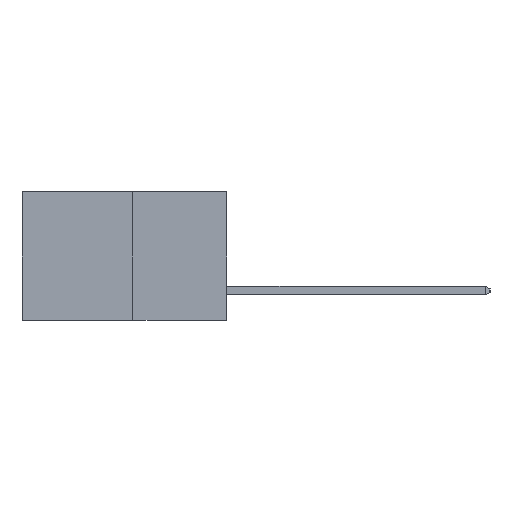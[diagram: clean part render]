
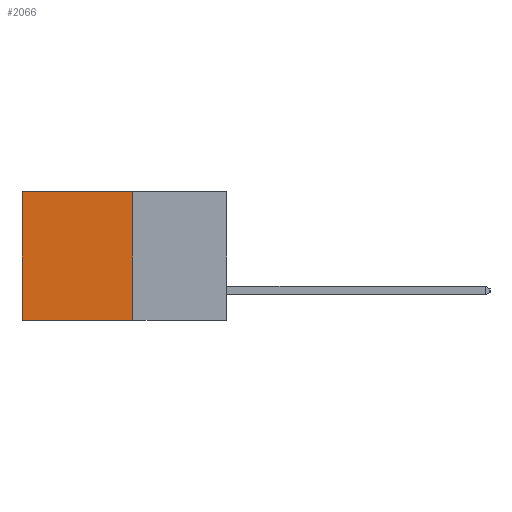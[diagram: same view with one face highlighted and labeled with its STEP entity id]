
A CAD part, left-side view. The second image highlights one B-rep face of the part: STEP entity #2066.
In plain terms, the highlighted planar face has unit normal (-1, 0, 0).
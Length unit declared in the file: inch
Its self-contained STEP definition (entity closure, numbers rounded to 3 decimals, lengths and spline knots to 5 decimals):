
#570 = VERTEX_POINT ( 'NONE', #11419 ) ;
#684 = EDGE_CURVE ( 'NONE', #3620, #5594, #8739, .T. ) ;
#844 = VECTOR ( 'NONE', #13764, 39.37008 ) ;
#1901 = PLANE ( 'NONE',  #9061 ) ;
#2066 = ADVANCED_FACE ( 'NONE', ( #10842 ), #1901, .F. ) ;
#2217 = EDGE_LOOP ( 'NONE', ( #8002, #12167, #5767, #13775 ) ) ;
#2970 = VERTEX_POINT ( 'NONE', #7666 ) ;
#3016 = EDGE_CURVE ( 'NONE', #570, #5594, #9937, .T. ) ;
#3083 = VECTOR ( 'NONE', #10998, 39.37008 ) ;
#3231 = CARTESIAN_POINT ( 'NONE',  ( 0.277, 0.27, 0. ) ) ;
#3547 = DIRECTION ( 'NONE',  ( 0., 0., -1. ) ) ;
#3620 = VERTEX_POINT ( 'NONE', #4545 ) ;
#3797 = LINE ( 'NONE', #3231, #12473 ) ;
#4545 = CARTESIAN_POINT ( 'NONE',  ( 0.277, 0.27, -0.37 ) ) ;
#4642 = LINE ( 'NONE', #8030, #844 ) ;
#5428 = EDGE_CURVE ( 'NONE', #2970, #570, #3797, .T. ) ;
#5594 = VERTEX_POINT ( 'NONE', #9767 ) ;
#5767 = ORIENTED_EDGE ( 'NONE', *, *, #13887, .F. ) ;
#7078 = DIRECTION ( 'NONE',  ( 0., 0., -1. ) ) ;
#7666 = CARTESIAN_POINT ( 'NONE',  ( 0.277, 0.27, 0. ) ) ;
#8002 = ORIENTED_EDGE ( 'NONE', *, *, #3016, .T. ) ;
#8030 = CARTESIAN_POINT ( 'NONE',  ( 0.277, 0.27, -0.37 ) ) ;
#8093 = CARTESIAN_POINT ( 'NONE',  ( 0.277, 0.27, -0.37 ) ) ;
#8477 = CARTESIAN_POINT ( 'NONE',  ( 0.277, 0.59, -0.37 ) ) ;
#8739 = LINE ( 'NONE', #8093, #3083 ) ;
#8903 = DIRECTION ( 'NONE',  ( 0., 1., 0. ) ) ;
#9061 = AXIS2_PLACEMENT_3D ( 'NONE', #13373, #11158, #3547 ) ;
#9567 = VECTOR ( 'NONE', #7078, 39.37008 ) ;
#9767 = CARTESIAN_POINT ( 'NONE',  ( 0.277, 0.59, -0.37 ) ) ;
#9937 = LINE ( 'NONE', #8477, #9567 ) ;
#10842 = FACE_OUTER_BOUND ( 'NONE', #2217, .T. ) ;
#10998 = DIRECTION ( 'NONE',  ( 0., 1., 0. ) ) ;
#11158 = DIRECTION ( 'NONE',  ( 1., 0., 0. ) ) ;
#11419 = CARTESIAN_POINT ( 'NONE',  ( 0.277, 0.59, 0. ) ) ;
#12167 = ORIENTED_EDGE ( 'NONE', *, *, #684, .F. ) ;
#12473 = VECTOR ( 'NONE', #8903, 39.37008 ) ;
#13373 = CARTESIAN_POINT ( 'NONE',  ( 0.277, 0.27, -0.37 ) ) ;
#13764 = DIRECTION ( 'NONE',  ( 0., 0., -1. ) ) ;
#13775 = ORIENTED_EDGE ( 'NONE', *, *, #5428, .T. ) ;
#13887 = EDGE_CURVE ( 'NONE', #2970, #3620, #4642, .T. ) ;
